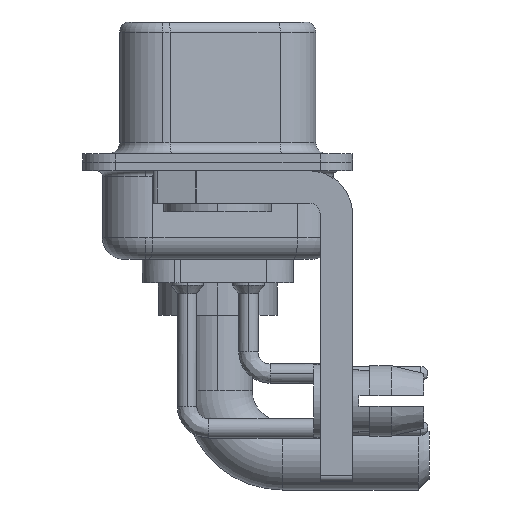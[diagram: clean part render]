
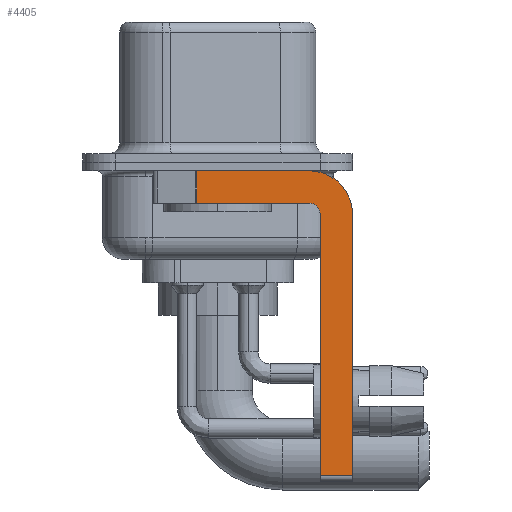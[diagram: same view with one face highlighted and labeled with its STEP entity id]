
A CAD part, left-side view. The second image highlights one B-rep face of the part: STEP entity #4405.
In plain terms, the highlighted planar face has unit normal (-1, 0, 0).
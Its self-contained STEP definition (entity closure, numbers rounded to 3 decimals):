
#49 = VERTEX_POINT ( 'NONE', #22412 ) ;
#1187 = VERTEX_POINT ( 'NONE', #18521 ) ;
#1792 = EDGE_CURVE ( 'NONE', #13811, #7295, #22389, .T. ) ;
#2007 = DIRECTION ( 'NONE',  ( 0., 0., -1. ) ) ;
#2047 = LINE ( 'NONE', #6179, #17351 ) ;
#2059 = DIRECTION ( 'NONE',  ( 0., -1., 0. ) ) ;
#2467 = EDGE_CURVE ( 'NONE', #13500, #12139, #8756, .T. ) ;
#2559 = DIRECTION ( 'NONE',  ( 0., 0., -1. ) ) ;
#2718 = DIRECTION ( 'NONE',  ( 0., -1., 0. ) ) ;
#2996 = CIRCLE ( 'NONE', #16989, 2. ) ;
#3345 = DIRECTION ( 'NONE',  ( 0., 0., 1. ) ) ;
#3846 = DIRECTION ( 'NONE',  ( 0., 1., 0. ) ) ;
#3897 = CARTESIAN_POINT ( 'NONE',  ( -2.9, -6.25, -2.4 ) ) ;
#4255 = CARTESIAN_POINT ( 'NONE',  ( -2.9, -4.25, -2.4 ) ) ;
#4405 = ADVANCED_FACE ( 'NONE', ( #9836 ), #4443, .F. ) ;
#4442 = DIRECTION ( 'NONE',  ( -1., 0., 0. ) ) ;
#4443 = PLANE ( 'NONE',  #12360 ) ;
#5117 = CARTESIAN_POINT ( 'NONE',  ( -2.9, -4.75, -14.8 ) ) ;
#5561 = CARTESIAN_POINT ( 'NONE',  ( -2.9, -4.75, -2.4 ) ) ;
#6179 = CARTESIAN_POINT ( 'NONE',  ( -2.9, 0.978, -1.9 ) ) ;
#6436 = VECTOR ( 'NONE', #2718, 1000. ) ;
#6495 = DIRECTION ( 'NONE',  ( 1., 0., 0. ) ) ;
#6591 = CIRCLE ( 'NONE', #15781, 0.5 ) ;
#6616 = VECTOR ( 'NONE', #3345, 1000. ) ;
#6632 = ORIENTED_EDGE ( 'NONE', *, *, #11813, .F. ) ;
#7097 = ORIENTED_EDGE ( 'NONE', *, *, #24559, .T. ) ;
#7295 = VERTEX_POINT ( 'NONE', #17602 ) ;
#7643 = VERTEX_POINT ( 'NONE', #10279 ) ;
#8199 = CARTESIAN_POINT ( 'NONE',  ( -2.9, -4.25, -2.4 ) ) ;
#8475 = LINE ( 'NONE', #10725, #6436 ) ;
#8756 = LINE ( 'NONE', #5117, #6616 ) ;
#9010 = VECTOR ( 'NONE', #3846, 1000. ) ;
#9299 = EDGE_CURVE ( 'NONE', #1187, #7295, #2047, .T. ) ;
#9836 = FACE_OUTER_BOUND ( 'NONE', #13895, .T. ) ;
#10074 = DIRECTION ( 'NONE',  ( 0., 0., 1. ) ) ;
#10200 = CARTESIAN_POINT ( 'NONE',  ( -2.9, 3., -0.4 ) ) ;
#10279 = CARTESIAN_POINT ( 'NONE',  ( -2.9, -4.25, -0.4 ) ) ;
#10479 = EDGE_CURVE ( 'NONE', #7643, #49, #2996, .T. ) ;
#10725 = CARTESIAN_POINT ( 'NONE',  ( -2.9, -4.25, -14.55 ) ) ;
#11231 = ORIENTED_EDGE ( 'NONE', *, *, #17478, .F. ) ;
#11813 = EDGE_CURVE ( 'NONE', #12139, #13811, #6591, .T. ) ;
#12124 = DIRECTION ( 'NONE',  ( 0., 0., -1. ) ) ;
#12139 = VERTEX_POINT ( 'NONE', #5561 ) ;
#12360 = AXIS2_PLACEMENT_3D ( 'NONE', #13706, #19724, #2559 ) ;
#12447 = ORIENTED_EDGE ( 'NONE', *, *, #9299, .T. ) ;
#13109 = CARTESIAN_POINT ( 'NONE',  ( -2.9, -4.25, -1.9 ) ) ;
#13395 = LINE ( 'NONE', #3897, #17039 ) ;
#13500 = VERTEX_POINT ( 'NONE', #14587 ) ;
#13706 = CARTESIAN_POINT ( 'NONE',  ( -2.9, -4.25, -2.4 ) ) ;
#13811 = VERTEX_POINT ( 'NONE', #17591 ) ;
#13895 = EDGE_LOOP ( 'NONE', ( #17228, #12447, #22823, #6632, #21585, #7097, #11231, #16566 ) ) ;
#14587 = CARTESIAN_POINT ( 'NONE',  ( -2.9, -4.75, -14.55 ) ) ;
#15140 = EDGE_CURVE ( 'NONE', #1187, #7643, #15966, .T. ) ;
#15781 = AXIS2_PLACEMENT_3D ( 'NONE', #8199, #4442, #10074 ) ;
#15813 = VECTOR ( 'NONE', #2059, 1000. ) ;
#15966 = LINE ( 'NONE', #10200, #15813 ) ;
#16566 = ORIENTED_EDGE ( 'NONE', *, *, #10479, .F. ) ;
#16989 = AXIS2_PLACEMENT_3D ( 'NONE', #4255, #6495, #12124 ) ;
#17039 = VECTOR ( 'NONE', #2007, 1000. ) ;
#17228 = ORIENTED_EDGE ( 'NONE', *, *, #15140, .F. ) ;
#17351 = VECTOR ( 'NONE', #21335, 1000. ) ;
#17478 = EDGE_CURVE ( 'NONE', #49, #20433, #13395, .T. ) ;
#17591 = CARTESIAN_POINT ( 'NONE',  ( -2.9, -4.25, -1.9 ) ) ;
#17602 = CARTESIAN_POINT ( 'NONE',  ( -2.9, 0.978, -1.9 ) ) ;
#18521 = CARTESIAN_POINT ( 'NONE',  ( -2.9, 0.978, -0.4 ) ) ;
#19724 = DIRECTION ( 'NONE',  ( 1., 0., 0. ) ) ;
#20433 = VERTEX_POINT ( 'NONE', #20790 ) ;
#20790 = CARTESIAN_POINT ( 'NONE',  ( -2.9, -6.25, -14.55 ) ) ;
#21335 = DIRECTION ( 'NONE',  ( 0., 0., -1. ) ) ;
#21585 = ORIENTED_EDGE ( 'NONE', *, *, #2467, .F. ) ;
#22389 = LINE ( 'NONE', #13109, #9010 ) ;
#22412 = CARTESIAN_POINT ( 'NONE',  ( -2.9, -6.25, -2.4 ) ) ;
#22823 = ORIENTED_EDGE ( 'NONE', *, *, #1792, .F. ) ;
#24559 = EDGE_CURVE ( 'NONE', #13500, #20433, #8475, .T. ) ;
